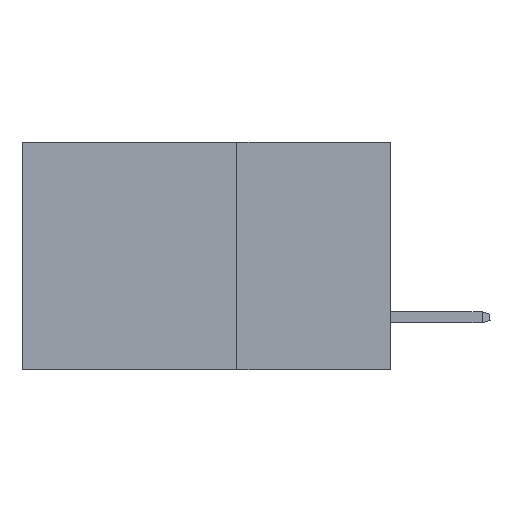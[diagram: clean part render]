
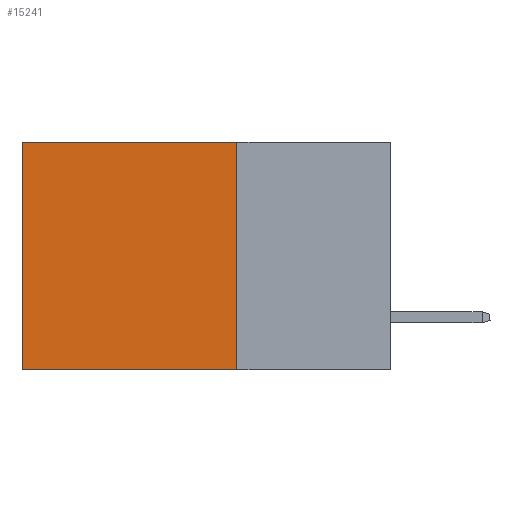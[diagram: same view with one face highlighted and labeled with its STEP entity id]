
A CAD part, left-side view. The second image highlights one B-rep face of the part: STEP entity #15241.
In plain terms, the highlighted planar face has unit normal (-1, 0, 0).
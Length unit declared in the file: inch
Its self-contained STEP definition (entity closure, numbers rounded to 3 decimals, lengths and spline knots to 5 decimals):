
#261 = VECTOR ( 'NONE', #14614, 39.37008 ) ;
#1185 = CARTESIAN_POINT ( 'NONE',  ( 0.2875, 0.6, 0. ) ) ;
#1244 = DIRECTION ( 'NONE',  ( 1., 0., 0. ) ) ;
#1552 = LINE ( 'NONE', #10792, #17325 ) ;
#1555 = VECTOR ( 'NONE', #11689, 39.37008 ) ;
#1619 = CARTESIAN_POINT ( 'NONE',  ( 0.2875, 0.25, -0.37 ) ) ;
#1973 = DIRECTION ( 'NONE',  ( 0., 1., 0. ) ) ;
#2016 = EDGE_LOOP ( 'NONE', ( #5677, #13605, #12223, #11204 ) ) ;
#2365 = VERTEX_POINT ( 'NONE', #1185 ) ;
#2690 = CARTESIAN_POINT ( 'NONE',  ( 0.2875, 0.25, 0. ) ) ;
#2849 = CARTESIAN_POINT ( 'NONE',  ( 0.2875, 0.6, 0. ) ) ;
#3280 = FACE_OUTER_BOUND ( 'NONE', #2016, .T. ) ;
#3580 = EDGE_CURVE ( 'NONE', #7992, #8619, #3963, .T. ) ;
#3963 = LINE ( 'NONE', #16953, #6856 ) ;
#4483 = LINE ( 'NONE', #1619, #1555 ) ;
#5677 = ORIENTED_EDGE ( 'NONE', *, *, #16896, .T. ) ;
#6770 = DIRECTION ( 'NONE',  ( 0., 0., -1. ) ) ;
#6856 = VECTOR ( 'NONE', #6770, 39.37008 ) ;
#6907 = VERTEX_POINT ( 'NONE', #17312 ) ;
#6924 = EDGE_CURVE ( 'NONE', #8619, #6907, #4483, .T. ) ;
#7992 = VERTEX_POINT ( 'NONE', #17067 ) ;
#8619 = VERTEX_POINT ( 'NONE', #12271 ) ;
#10268 = EDGE_CURVE ( 'NONE', #7992, #2365, #1552, .T. ) ;
#10792 = CARTESIAN_POINT ( 'NONE',  ( 0.2875, 0.25, 0. ) ) ;
#11204 = ORIENTED_EDGE ( 'NONE', *, *, #10268, .T. ) ;
#11689 = DIRECTION ( 'NONE',  ( 0., 1., 0. ) ) ;
#12223 = ORIENTED_EDGE ( 'NONE', *, *, #3580, .F. ) ;
#12271 = CARTESIAN_POINT ( 'NONE',  ( 0.2875, 0.25, -0.37 ) ) ;
#12777 = DIRECTION ( 'NONE',  ( 0., 0., -1. ) ) ;
#13347 = LINE ( 'NONE', #2849, #261 ) ;
#13605 = ORIENTED_EDGE ( 'NONE', *, *, #6924, .F. ) ;
#14614 = DIRECTION ( 'NONE',  ( 0., 0., -1. ) ) ;
#15241 = ADVANCED_FACE ( 'NONE', ( #3280 ), #15580, .F. ) ;
#15580 = PLANE ( 'NONE',  #16799 ) ;
#16799 = AXIS2_PLACEMENT_3D ( 'NONE', #2690, #1244, #12777 ) ;
#16896 = EDGE_CURVE ( 'NONE', #2365, #6907, #13347, .T. ) ;
#16953 = CARTESIAN_POINT ( 'NONE',  ( 0.2875, 0.25, 0. ) ) ;
#17067 = CARTESIAN_POINT ( 'NONE',  ( 0.2875, 0.25, 0. ) ) ;
#17312 = CARTESIAN_POINT ( 'NONE',  ( 0.2875, 0.6, -0.37 ) ) ;
#17325 = VECTOR ( 'NONE', #1973, 39.37008 ) ;
